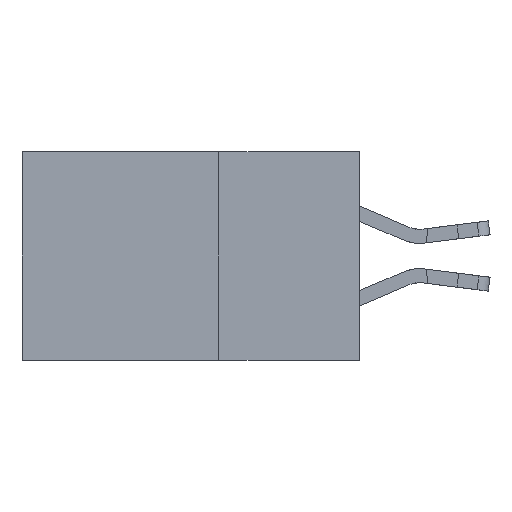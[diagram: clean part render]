
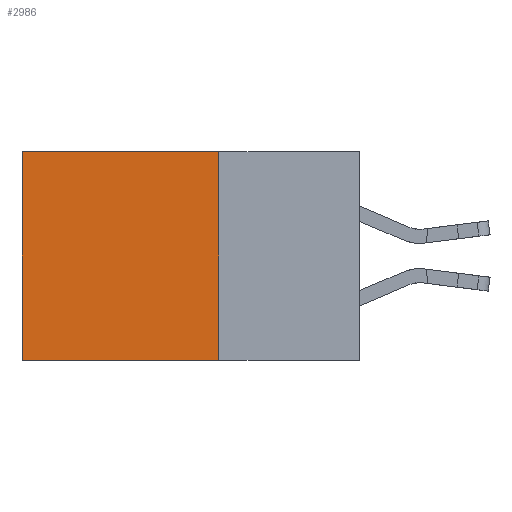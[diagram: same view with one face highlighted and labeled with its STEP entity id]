
A CAD part, left-side view. The second image highlights one B-rep face of the part: STEP entity #2986.
In plain terms, the highlighted planar face has unit normal (-1, 0, 0).
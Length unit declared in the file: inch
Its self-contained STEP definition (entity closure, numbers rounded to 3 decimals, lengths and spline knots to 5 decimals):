
#1309 = LINE ( 'NONE', #11267, #18981 ) ;
#1532 = VECTOR ( 'NONE', #10412, 39.37008 ) ;
#1750 = ORIENTED_EDGE ( 'NONE', *, *, #11959, .T. ) ;
#2062 = LINE ( 'NONE', #9977, #11343 ) ;
#2439 = EDGE_CURVE ( 'NONE', #9758, #11890, #19038, .T. ) ;
#2620 = CARTESIAN_POINT ( 'NONE',  ( 0.2875, 0.6, -0.37 ) ) ;
#2986 = ADVANCED_FACE ( 'NONE', ( #16068 ), #10901, .F. ) ;
#3224 = ORIENTED_EDGE ( 'NONE', *, *, #8820, .T. ) ;
#3243 = DIRECTION ( 'NONE',  ( 0., 0., -1. ) ) ;
#3653 = VECTOR ( 'NONE', #9047, 39.37008 ) ;
#4520 = CARTESIAN_POINT ( 'NONE',  ( 0.2875, 0.25, 0. ) ) ;
#5317 = CARTESIAN_POINT ( 'NONE',  ( 0.2875, 0.25, -0.37 ) ) ;
#5819 = DIRECTION ( 'NONE',  ( 1., 0., 0. ) ) ;
#7256 = ORIENTED_EDGE ( 'NONE', *, *, #2439, .F. ) ;
#8820 = EDGE_CURVE ( 'NONE', #17104, #11890, #1309, .T. ) ;
#9047 = DIRECTION ( 'NONE',  ( 0., 1., 0. ) ) ;
#9758 = VERTEX_POINT ( 'NONE', #5317 ) ;
#9774 = DIRECTION ( 'NONE',  ( 0., 1., 0. ) ) ;
#9977 = CARTESIAN_POINT ( 'NONE',  ( 0.2875, 0.25, 0. ) ) ;
#10305 = DIRECTION ( 'NONE',  ( 0., 0., -1. ) ) ;
#10412 = DIRECTION ( 'NONE',  ( 0., 0., -1. ) ) ;
#10901 = PLANE ( 'NONE',  #13614 ) ;
#11267 = CARTESIAN_POINT ( 'NONE',  ( 0.2875, 0.6, 0. ) ) ;
#11343 = VECTOR ( 'NONE', #9774, 39.37008 ) ;
#11698 = EDGE_CURVE ( 'NONE', #12090, #9758, #17392, .T. ) ;
#11890 = VERTEX_POINT ( 'NONE', #2620 ) ;
#11959 = EDGE_CURVE ( 'NONE', #12090, #17104, #2062, .T. ) ;
#12090 = VERTEX_POINT ( 'NONE', #12737 ) ;
#12737 = CARTESIAN_POINT ( 'NONE',  ( 0.2875, 0.25, 0. ) ) ;
#12901 = CARTESIAN_POINT ( 'NONE',  ( 0.2875, 0.6, 0. ) ) ;
#13614 = AXIS2_PLACEMENT_3D ( 'NONE', #4520, #5819, #3243 ) ;
#13789 = CARTESIAN_POINT ( 'NONE',  ( 0.2875, 0.25, -0.37 ) ) ;
#16068 = FACE_OUTER_BOUND ( 'NONE', #16783, .T. ) ;
#16783 = EDGE_LOOP ( 'NONE', ( #3224, #7256, #20255, #1750 ) ) ;
#17104 = VERTEX_POINT ( 'NONE', #12901 ) ;
#17392 = LINE ( 'NONE', #20219, #1532 ) ;
#18981 = VECTOR ( 'NONE', #10305, 39.37008 ) ;
#19038 = LINE ( 'NONE', #13789, #3653 ) ;
#20219 = CARTESIAN_POINT ( 'NONE',  ( 0.2875, 0.25, 0. ) ) ;
#20255 = ORIENTED_EDGE ( 'NONE', *, *, #11698, .F. ) ;
